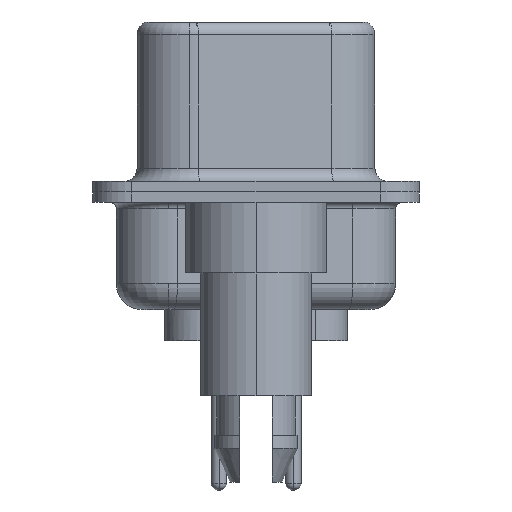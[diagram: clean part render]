
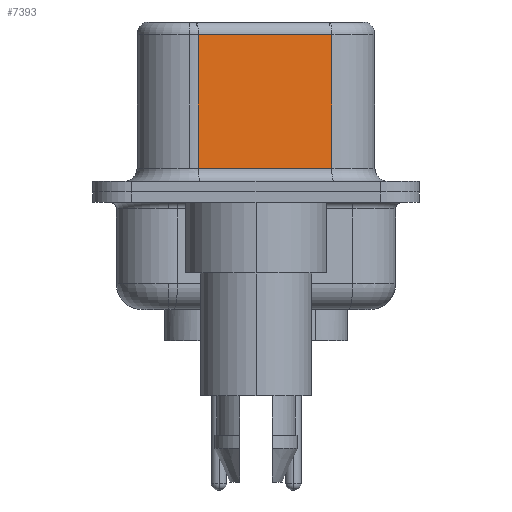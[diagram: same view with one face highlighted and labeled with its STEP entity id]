
A CAD part, left-side view. The second image highlights one B-rep face of the part: STEP entity #7393.
In plain terms, the highlighted planar face has unit normal (-0.985, -0.174, 0).
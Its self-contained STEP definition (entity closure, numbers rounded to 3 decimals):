
#148 = DIRECTION ( 'NONE',  ( 0., 0., -1. ) ) ;
#1517 = AXIS2_PLACEMENT_3D ( 'NONE', #5434, #13478, #21194 ) ;
#1552 = CARTESIAN_POINT ( 'NONE',  ( 3.68, 2.203, 6.02 ) ) ;
#1740 = LINE ( 'NONE', #9910, #11578 ) ;
#2552 = CARTESIAN_POINT ( 'NONE',  ( 4.58, -2.897, 6.02 ) ) ;
#2694 = EDGE_LOOP ( 'NONE', ( #23794, #17152, #13074, #6841 ) ) ;
#2708 = VECTOR ( 'NONE', #148, 1000. ) ;
#3712 = DIRECTION ( 'NONE',  ( 0.174, -0.985, 0. ) ) ;
#4789 = LINE ( 'NONE', #2552, #14963 ) ;
#4840 = EDGE_CURVE ( 'NONE', #19952, #7933, #8055, .T. ) ;
#5434 = CARTESIAN_POINT ( 'NONE',  ( 4.58, -2.897, 6.52 ) ) ;
#5786 = EDGE_CURVE ( 'NONE', #7820, #19952, #4789, .T. ) ;
#6767 = DIRECTION ( 'NONE',  ( -0.174, 0.985, 0. ) ) ;
#6841 = ORIENTED_EDGE ( 'NONE', *, *, #22050, .T. ) ;
#7393 = ADVANCED_FACE ( 'NONE', ( #13086 ), #9129, .F. ) ;
#7820 = VERTEX_POINT ( 'NONE', #18931 ) ;
#7933 = VERTEX_POINT ( 'NONE', #16971 ) ;
#8055 = LINE ( 'NONE', #15961, #24116 ) ;
#9129 = PLANE ( 'NONE',  #1517 ) ;
#9910 = CARTESIAN_POINT ( 'NONE',  ( 4.58, -2.897, 0.9 ) ) ;
#11578 = VECTOR ( 'NONE', #3712, 1000. ) ;
#11882 = DIRECTION ( 'NONE',  ( 0., 0., -1. ) ) ;
#12869 = VERTEX_POINT ( 'NONE', #21551 ) ;
#13074 = ORIENTED_EDGE ( 'NONE', *, *, #4840, .T. ) ;
#13086 = FACE_OUTER_BOUND ( 'NONE', #2694, .T. ) ;
#13478 = DIRECTION ( 'NONE',  ( 0.985, 0.174, 0. ) ) ;
#14137 = LINE ( 'NONE', #23953, #2708 ) ;
#14963 = VECTOR ( 'NONE', #6767, 1000. ) ;
#15961 = CARTESIAN_POINT ( 'NONE',  ( 3.68, 2.203, 6.52 ) ) ;
#16971 = CARTESIAN_POINT ( 'NONE',  ( 3.68, 2.203, 0.9 ) ) ;
#17152 = ORIENTED_EDGE ( 'NONE', *, *, #5786, .T. ) ;
#18931 = CARTESIAN_POINT ( 'NONE',  ( 4.58, -2.897, 6.02 ) ) ;
#19952 = VERTEX_POINT ( 'NONE', #1552 ) ;
#21194 = DIRECTION ( 'NONE',  ( -0.174, 0.985, 0. ) ) ;
#21551 = CARTESIAN_POINT ( 'NONE',  ( 4.58, -2.897, 0.9 ) ) ;
#22050 = EDGE_CURVE ( 'NONE', #7933, #12869, #1740, .T. ) ;
#23794 = ORIENTED_EDGE ( 'NONE', *, *, #25065, .F. ) ;
#23953 = CARTESIAN_POINT ( 'NONE',  ( 4.58, -2.897, 6.52 ) ) ;
#24116 = VECTOR ( 'NONE', #11882, 1000. ) ;
#25065 = EDGE_CURVE ( 'NONE', #7820, #12869, #14137, .T. ) ;
